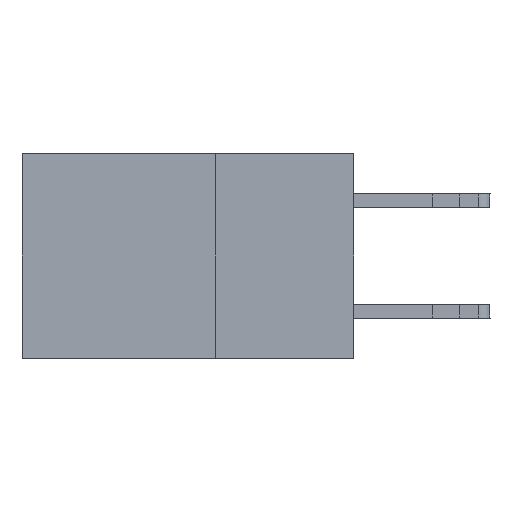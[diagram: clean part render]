
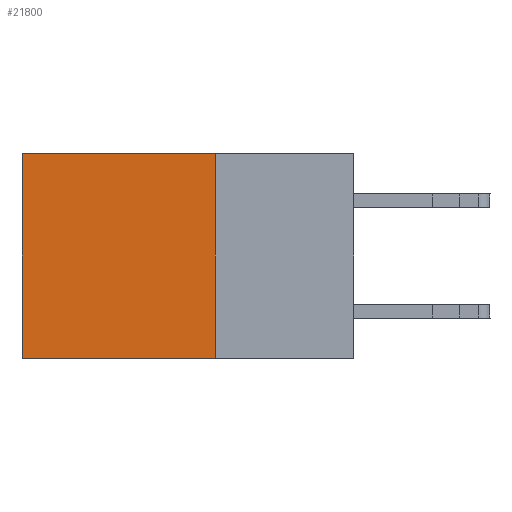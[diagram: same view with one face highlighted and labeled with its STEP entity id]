
A CAD part, left-side view. The second image highlights one B-rep face of the part: STEP entity #21800.
In plain terms, the highlighted planar face has unit normal (-1, 0, 0).
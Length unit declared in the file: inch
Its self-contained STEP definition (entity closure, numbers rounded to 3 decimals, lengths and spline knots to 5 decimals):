
#664 = CARTESIAN_POINT ( 'NONE',  ( 0.2875, 0.25, 0. ) ) ;
#2004 = VECTOR ( 'NONE', #33103, 39.37008 ) ;
#4827 = ORIENTED_EDGE ( 'NONE', *, *, #22897, .T. ) ;
#4919 = EDGE_CURVE ( 'NONE', #12500, #37038, #31327, .T. ) ;
#5974 = CARTESIAN_POINT ( 'NONE',  ( 0.2875, 0.25, -0.37 ) ) ;
#6943 = FACE_OUTER_BOUND ( 'NONE', #26828, .T. ) ;
#7085 = CARTESIAN_POINT ( 'NONE',  ( 0.2875, 0.6, 0. ) ) ;
#7171 = CARTESIAN_POINT ( 'NONE',  ( 0.2875, 0.6, -0.37 ) ) ;
#12500 = VERTEX_POINT ( 'NONE', #25674 ) ;
#12845 = AXIS2_PLACEMENT_3D ( 'NONE', #18434, #30354, #18570 ) ;
#14097 = DIRECTION ( 'NONE',  ( 0., 0., -1. ) ) ;
#14592 = VECTOR ( 'NONE', #34152, 39.37008 ) ;
#16797 = VECTOR ( 'NONE', #14097, 39.37008 ) ;
#18340 = CARTESIAN_POINT ( 'NONE',  ( 0.2875, 0.6, 0. ) ) ;
#18434 = CARTESIAN_POINT ( 'NONE',  ( 0.2875, 0.25, 0. ) ) ;
#18570 = DIRECTION ( 'NONE',  ( 0., 0., -1. ) ) ;
#18812 = VERTEX_POINT ( 'NONE', #18340 ) ;
#19658 = VERTEX_POINT ( 'NONE', #7171 ) ;
#20504 = CARTESIAN_POINT ( 'NONE',  ( 0.2875, 0.25, 0. ) ) ;
#21800 = ADVANCED_FACE ( 'NONE', ( #6943 ), #30601, .F. ) ;
#22097 = LINE ( 'NONE', #664, #2004 ) ;
#22897 = EDGE_CURVE ( 'NONE', #12500, #18812, #22097, .T. ) ;
#23817 = CARTESIAN_POINT ( 'NONE',  ( 0.2875, 0.25, -0.37 ) ) ;
#24716 = EDGE_CURVE ( 'NONE', #37038, #19658, #28121, .T. ) ;
#25674 = CARTESIAN_POINT ( 'NONE',  ( 0.2875, 0.25, 0. ) ) ;
#26828 = EDGE_LOOP ( 'NONE', ( #30944, #28683, #27473, #4827 ) ) ;
#27473 = ORIENTED_EDGE ( 'NONE', *, *, #4919, .F. ) ;
#28121 = LINE ( 'NONE', #23817, #38424 ) ;
#28683 = ORIENTED_EDGE ( 'NONE', *, *, #24716, .F. ) ;
#30354 = DIRECTION ( 'NONE',  ( 1., 0., 0. ) ) ;
#30601 = PLANE ( 'NONE',  #12845 ) ;
#30944 = ORIENTED_EDGE ( 'NONE', *, *, #34937, .T. ) ;
#31327 = LINE ( 'NONE', #20504, #16797 ) ;
#33103 = DIRECTION ( 'NONE',  ( 0., 1., 0. ) ) ;
#33770 = LINE ( 'NONE', #7085, #14592 ) ;
#34152 = DIRECTION ( 'NONE',  ( 0., 0., -1. ) ) ;
#34937 = EDGE_CURVE ( 'NONE', #18812, #19658, #33770, .T. ) ;
#35727 = DIRECTION ( 'NONE',  ( 0., 1., 0. ) ) ;
#37038 = VERTEX_POINT ( 'NONE', #5974 ) ;
#38424 = VECTOR ( 'NONE', #35727, 39.37008 ) ;
